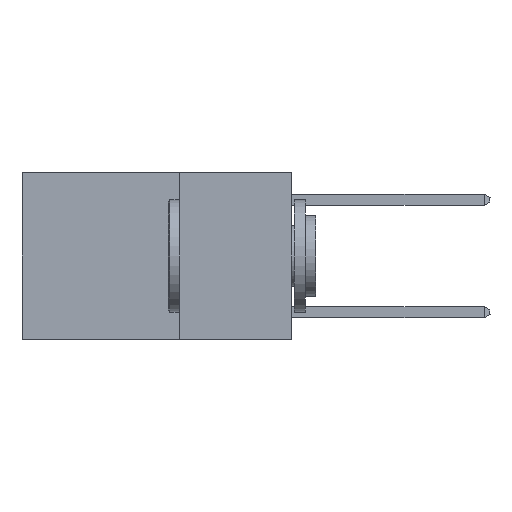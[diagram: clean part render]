
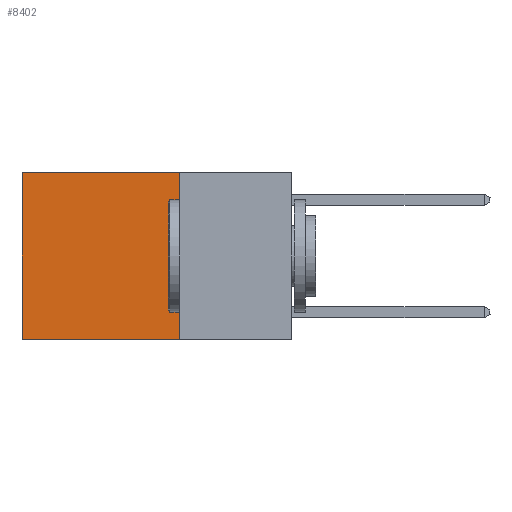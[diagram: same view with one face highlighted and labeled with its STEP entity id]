
A CAD part, left-side view. The second image highlights one B-rep face of the part: STEP entity #8402.
In plain terms, the highlighted planar face has unit normal (-1, 0, 0).
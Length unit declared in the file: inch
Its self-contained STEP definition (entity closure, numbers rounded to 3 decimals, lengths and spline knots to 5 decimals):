
#277 = VECTOR ( 'NONE', #10639, 39.37008 ) ;
#280 = DIRECTION ( 'NONE',  ( 1., 0., 0. ) ) ;
#787 = VECTOR ( 'NONE', #5193, 39.37008 ) ;
#1295 = LINE ( 'NONE', #8007, #277 ) ;
#1482 = ORIENTED_EDGE ( 'NONE', *, *, #9963, .F. ) ;
#1859 = VERTEX_POINT ( 'NONE', #8804 ) ;
#1917 = ORIENTED_EDGE ( 'NONE', *, *, #2107, .T. ) ;
#2107 = EDGE_CURVE ( 'NONE', #8902, #1859, #9373, .T. ) ;
#2163 = CARTESIAN_POINT ( 'NONE',  ( 0.2625, 0.25, 0. ) ) ;
#2538 = CARTESIAN_POINT ( 'NONE',  ( 0.2625, 0.25, 0. ) ) ;
#2688 = LINE ( 'NONE', #3414, #2761 ) ;
#2761 = VECTOR ( 'NONE', #7679, 39.37008 ) ;
#3286 = VERTEX_POINT ( 'NONE', #8360 ) ;
#3358 = CARTESIAN_POINT ( 'NONE',  ( 0.2625, 0.6, -0.37 ) ) ;
#3383 = EDGE_LOOP ( 'NONE', ( #6698, #1482, #10810, #1917 ) ) ;
#3390 = EDGE_CURVE ( 'NONE', #1859, #6744, #5306, .T. ) ;
#3414 = CARTESIAN_POINT ( 'NONE',  ( 0.2625, 0.25, 0. ) ) ;
#3429 = VECTOR ( 'NONE', #3666, 39.37008 ) ;
#3666 = DIRECTION ( 'NONE',  ( 0., 1., 0. ) ) ;
#3942 = EDGE_CURVE ( 'NONE', #8902, #3286, #2688, .T. ) ;
#4513 = DIRECTION ( 'NONE',  ( 0., 0., -1. ) ) ;
#5193 = DIRECTION ( 'NONE',  ( 0., 0., -1. ) ) ;
#5218 = CARTESIAN_POINT ( 'NONE',  ( 0.2625, 0.25, 0. ) ) ;
#5300 = AXIS2_PLACEMENT_3D ( 'NONE', #2538, #280, #4513 ) ;
#5306 = LINE ( 'NONE', #5921, #787 ) ;
#5921 = CARTESIAN_POINT ( 'NONE',  ( 0.2625, 0.6, 0. ) ) ;
#6698 = ORIENTED_EDGE ( 'NONE', *, *, #3390, .T. ) ;
#6744 = VERTEX_POINT ( 'NONE', #3358 ) ;
#7679 = DIRECTION ( 'NONE',  ( 0., 0., -1. ) ) ;
#8007 = CARTESIAN_POINT ( 'NONE',  ( 0.2625, 0.25, -0.37 ) ) ;
#8360 = CARTESIAN_POINT ( 'NONE',  ( 0.2625, 0.25, -0.37 ) ) ;
#8402 = ADVANCED_FACE ( 'NONE', ( #10885 ), #10047, .F. ) ;
#8804 = CARTESIAN_POINT ( 'NONE',  ( 0.2625, 0.6, 0. ) ) ;
#8902 = VERTEX_POINT ( 'NONE', #2163 ) ;
#9373 = LINE ( 'NONE', #5218, #3429 ) ;
#9963 = EDGE_CURVE ( 'NONE', #3286, #6744, #1295, .T. ) ;
#10047 = PLANE ( 'NONE',  #5300 ) ;
#10639 = DIRECTION ( 'NONE',  ( 0., 1., 0. ) ) ;
#10810 = ORIENTED_EDGE ( 'NONE', *, *, #3942, .F. ) ;
#10885 = FACE_OUTER_BOUND ( 'NONE', #3383, .T. ) ;
